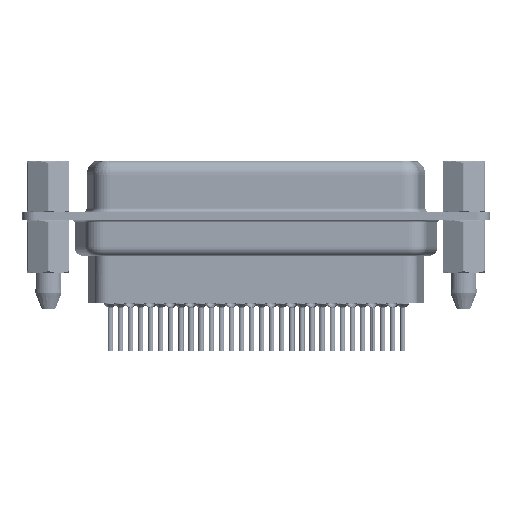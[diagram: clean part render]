
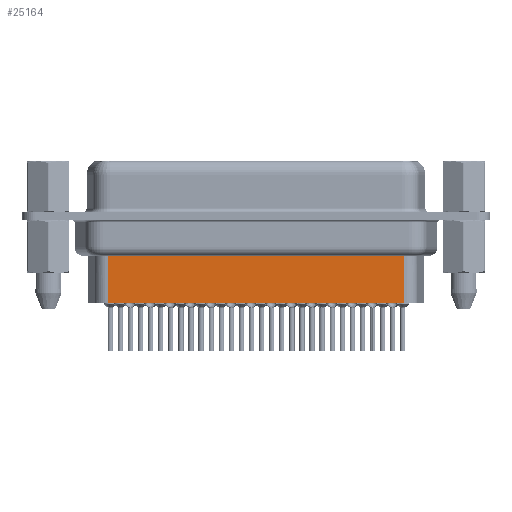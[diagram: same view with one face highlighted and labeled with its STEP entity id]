
A CAD part, front view. The second image highlights one B-rep face of the part: STEP entity #25164.
In plain terms, the highlighted planar face has unit normal (0, -1, 0).
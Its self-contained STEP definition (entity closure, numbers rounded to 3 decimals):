
#218 = CARTESIAN_POINT ( 'NONE',  ( 6.701, -3.5, -3.1 ) ) ;
#381 = AXIS2_PLACEMENT_3D ( 'NONE', #218, #28726, #39325 ) ;
#2718 = EDGE_CURVE ( 'NONE', #21820, #11050, #8751, .T. ) ;
#4121 = DIRECTION ( 'NONE',  ( -1., 0., 0. ) ) ;
#7262 = DIRECTION ( 'NONE',  ( 0., 0., -1. ) ) ;
#7489 = CARTESIAN_POINT ( 'NONE',  ( 6.701, -3.5, -3.1 ) ) ;
#8751 = LINE ( 'NONE', #20116, #16005 ) ;
#10555 = ORIENTED_EDGE ( 'NONE', *, *, #2718, .T. ) ;
#11050 = VERTEX_POINT ( 'NONE', #19428 ) ;
#11735 = EDGE_CURVE ( 'NONE', #30377, #20914, #32367, .T. ) ;
#12538 = EDGE_CURVE ( 'NONE', #11050, #20914, #21195, .T. ) ;
#14841 = ORIENTED_EDGE ( 'NONE', *, *, #18055, .F. ) ;
#15866 = EDGE_LOOP ( 'NONE', ( #14841, #10555, #26752, #22253 ) ) ;
#16005 = VECTOR ( 'NONE', #40177, 1000. ) ;
#17433 = CARTESIAN_POINT ( 'NONE',  ( 40.339, -3.5, -3.1 ) ) ;
#18055 = EDGE_CURVE ( 'NONE', #21820, #30377, #31083, .T. ) ;
#19428 = CARTESIAN_POINT ( 'NONE',  ( 6.701, -3.5, -4.097 ) ) ;
#20116 = CARTESIAN_POINT ( 'NONE',  ( 6.454, -3.5, -4.097 ) ) ;
#20914 = VERTEX_POINT ( 'NONE', #44280 ) ;
#20929 = DIRECTION ( 'NONE',  ( 0., 0., -1. ) ) ;
#21195 = LINE ( 'NONE', #7489, #28532 ) ;
#21820 = VERTEX_POINT ( 'NONE', #29582 ) ;
#22253 = ORIENTED_EDGE ( 'NONE', *, *, #11735, .F. ) ;
#25164 = ADVANCED_FACE ( 'NONE', ( #28050 ), #31961, .T. ) ;
#26752 = ORIENTED_EDGE ( 'NONE', *, *, #12538, .T. ) ;
#28050 = FACE_OUTER_BOUND ( 'NONE', #15866, .T. ) ;
#28532 = VECTOR ( 'NONE', #7262, 1000. ) ;
#28726 = DIRECTION ( 'NONE',  ( 0., -1., 0. ) ) ;
#29582 = CARTESIAN_POINT ( 'NONE',  ( 40.339, -3.5, -4.097 ) ) ;
#30222 = VECTOR ( 'NONE', #20929, 1000. ) ;
#30377 = VERTEX_POINT ( 'NONE', #43372 ) ;
#30656 = VECTOR ( 'NONE', #4121, 1000. ) ;
#31083 = LINE ( 'NONE', #17433, #30222 ) ;
#31961 = PLANE ( 'NONE',  #381 ) ;
#32367 = LINE ( 'NONE', #43437, #30656 ) ;
#39325 = DIRECTION ( 'NONE',  ( 1., 0., 0. ) ) ;
#40177 = DIRECTION ( 'NONE',  ( -1., 0., 0. ) ) ;
#43372 = CARTESIAN_POINT ( 'NONE',  ( 40.339, -3.5, -9.85 ) ) ;
#43437 = CARTESIAN_POINT ( 'NONE',  ( 6.701, -3.5, -9.85 ) ) ;
#44280 = CARTESIAN_POINT ( 'NONE',  ( 6.701, -3.5, -9.85 ) ) ;
